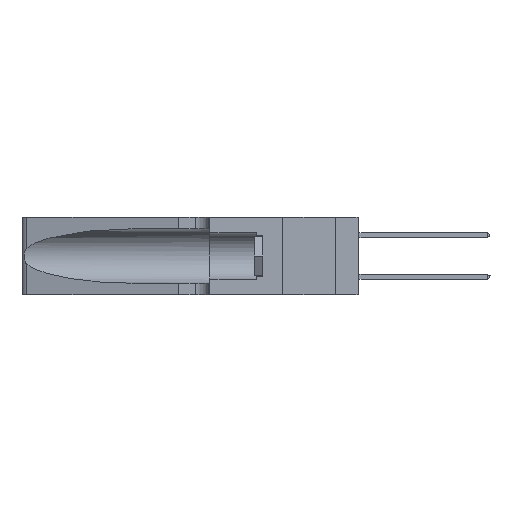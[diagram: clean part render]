
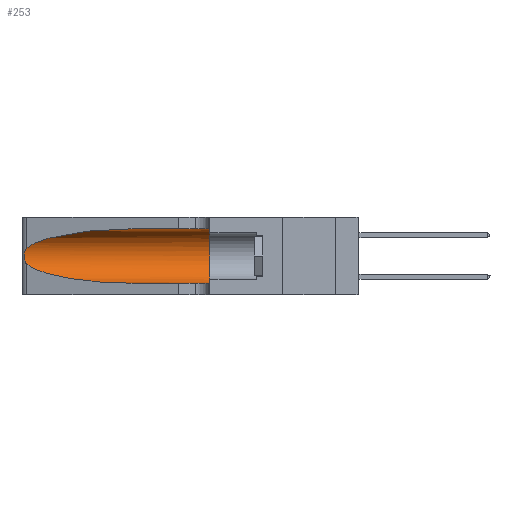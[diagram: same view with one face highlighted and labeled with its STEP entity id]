
A CAD part, left-side view. The second image highlights one B-rep face of the part: STEP entity #253.
In plain terms, the highlighted cylindrical face has radius 3.308 mm (diameter 6.617 mm), a partial arc.
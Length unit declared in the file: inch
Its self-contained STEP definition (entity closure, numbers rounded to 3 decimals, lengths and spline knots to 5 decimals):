
#198 = EDGE_CURVE ( 'NONE', #13411, #4651, #29645, .T. ) ;
#253 = ADVANCED_FACE ( 'NONE', ( #21866 ), #13304, .F. ) ;
#321 = DIRECTION ( 'NONE',  ( 0., 0., -1. ) ) ;
#993 = EDGE_CURVE ( 'NONE', #29057, #10696, #4352, .T. ) ;
#1692 = LINE ( 'NONE', #2280, #30447 ) ;
#2112 = CARTESIAN_POINT ( 'NONE',  ( 0.25487, 1.22718, 0.14631 ) ) ;
#2280 = CARTESIAN_POINT ( 'NONE',  ( 0.1305, 1.61858, 0.05475 ) ) ;
#2541 = CARTESIAN_POINT ( 'NONE',  ( 0.1305, 0.35, 0.185 ) ) ;
#2938 = VERTEX_POINT ( 'NONE', #15680 ) ;
#3268 =( BOUNDED_CURVE ( )  B_SPLINE_CURVE ( 3, ( #12375, #4944, #30703, #20521 ),
 .UNSPECIFIED., .F., .F. ) 
 B_SPLINE_CURVE_WITH_KNOTS ( ( 4, 4 ),
 ( 1.5708, 2.84003 ),
 .UNSPECIFIED. ) 
 CURVE ( )  GEOMETRIC_REPRESENTATION_ITEM ( )  RATIONAL_B_SPLINE_CURVE ( ( 1., 0.87, 0.87, 1. ) ) 
 REPRESENTATION_ITEM ( '' )  );
#4018 = ORIENTED_EDGE ( 'NONE', *, *, #198, .F. ) ;
#4308 = CARTESIAN_POINT ( 'NONE',  ( 0.1305, 0.72297, 0.05475 ) ) ;
#4352 = B_SPLINE_CURVE_WITH_KNOTS ( 'NONE', 3,
 ( #29398, #29007, #20638, #8054, #11064, #17375, #7347, #25163, #14851, #28022, #33294, #7217, #13134, #15459 ),
 .UNSPECIFIED., .F., .F.,
 ( 4, 2, 2, 2, 2, 2, 4 ),
 ( 0., 0.00027, 0.00053, 0.00107, 0.0016, 0.00187, 0.00214 ),
 .UNSPECIFIED. ) ;
#4651 = VERTEX_POINT ( 'NONE', #15916 ) ;
#4819 = DIRECTION ( 'NONE',  ( 0., -1., 0. ) ) ;
#4944 = CARTESIAN_POINT ( 'NONE',  ( 0.18966, 0.96281, 0.31525 ) ) ;
#4966 = DIRECTION ( 'NONE',  ( 0., 0., 1. ) ) ;
#5296 = CARTESIAN_POINT ( 'NONE',  ( 0.25487, 1.22718, 0.22369 ) ) ;
#5901 = EDGE_LOOP ( 'NONE', ( #16968, #30369, #29658, #20630, #4018, #18480 ) ) ;
#6521 = DIRECTION ( 'NONE',  ( 0., -1., 0. ) ) ;
#6953 = VERTEX_POINT ( 'NONE', #18798 ) ;
#7217 = CARTESIAN_POINT ( 'NONE',  ( 0.25639, 1.23186, 0.15144 ) ) ;
#7347 = CARTESIAN_POINT ( 'NONE',  ( 0.26075, 1.23896, 0.19203 ) ) ;
#7474 = EDGE_CURVE ( 'NONE', #6953, #29057, #3268, .T. ) ;
#8054 = CARTESIAN_POINT ( 'NONE',  ( 0.25787, 1.23484, 0.2124 ) ) ;
#8630 = CARTESIAN_POINT ( 'NONE',  ( 0.1305, 1.61858, 0.185 ) ) ;
#10174 = LINE ( 'NONE', #22243, #12628 ) ;
#10696 = VERTEX_POINT ( 'NONE', #2112 ) ;
#11064 = CARTESIAN_POINT ( 'NONE',  ( 0.25854, 1.2359, 0.20912 ) ) ;
#11968 = AXIS2_PLACEMENT_3D ( 'NONE', #2541, #12883, #4966 ) ;
#12375 = CARTESIAN_POINT ( 'NONE',  ( 0.1305, 0.72297, 0.31525 ) ) ;
#12628 = VECTOR ( 'NONE', #6521, 39.37008 ) ;
#12883 = DIRECTION ( 'NONE',  ( 0., 1., 0. ) ) ;
#13134 = CARTESIAN_POINT ( 'NONE',  ( 0.25555, 1.22993, 0.14849 ) ) ;
#13304 = CYLINDRICAL_SURFACE ( 'NONE', #29947, 0.13025 ) ;
#13411 = VERTEX_POINT ( 'NONE', #27493 ) ;
#14508 = EDGE_CURVE ( 'NONE', #10696, #2938, #22195, .T. ) ;
#14851 = CARTESIAN_POINT ( 'NONE',  ( 0.26017, 1.23833, 0.17102 ) ) ;
#15459 = CARTESIAN_POINT ( 'NONE',  ( 0.25487, 1.22718, 0.14631 ) ) ;
#15680 = CARTESIAN_POINT ( 'NONE',  ( 0.1305, 0.72297, 0.05475 ) ) ;
#15916 = CARTESIAN_POINT ( 'NONE',  ( 0.1305, 0.35, 0.05475 ) ) ;
#16550 = EDGE_CURVE ( 'NONE', #6953, #13411, #10174, .T. ) ;
#16798 = CARTESIAN_POINT ( 'NONE',  ( 0.25487, 1.22718, 0.14631 ) ) ;
#16968 = ORIENTED_EDGE ( 'NONE', *, *, #7474, .T. ) ;
#17375 = CARTESIAN_POINT ( 'NONE',  ( 0.26018, 1.23835, 0.19895 ) ) ;
#18480 = ORIENTED_EDGE ( 'NONE', *, *, #16550, .F. ) ;
#18798 = CARTESIAN_POINT ( 'NONE',  ( 0.1305, 0.72297, 0.31525 ) ) ;
#20521 = CARTESIAN_POINT ( 'NONE',  ( 0.25487, 1.22718, 0.22369 ) ) ;
#20630 = ORIENTED_EDGE ( 'NONE', *, *, #26491, .T. ) ;
#20638 = CARTESIAN_POINT ( 'NONE',  ( 0.25639, 1.23184, 0.21858 ) ) ;
#21866 = FACE_OUTER_BOUND ( 'NONE', #5901, .T. ) ;
#22195 =( BOUNDED_CURVE ( )  B_SPLINE_CURVE ( 3, ( #16798, #24346, #30562, #4308 ),
 .UNSPECIFIED., .F., .F. ) 
 B_SPLINE_CURVE_WITH_KNOTS ( ( 4, 4 ),
 ( 3.44316, 4.71239 ),
 .UNSPECIFIED. ) 
 CURVE ( )  GEOMETRIC_REPRESENTATION_ITEM ( )  RATIONAL_B_SPLINE_CURVE ( ( 1., 0.87, 0.87, 1. ) ) 
 REPRESENTATION_ITEM ( '' )  );
#22243 = CARTESIAN_POINT ( 'NONE',  ( 0.1305, 1.61858, 0.31525 ) ) ;
#23882 = DIRECTION ( 'NONE',  ( 0., -1., 0. ) ) ;
#24346 = CARTESIAN_POINT ( 'NONE',  ( 0.2373, 1.15595, 0.08982 ) ) ;
#25163 = CARTESIAN_POINT ( 'NONE',  ( 0.26075, 1.23896, 0.178 ) ) ;
#26491 = EDGE_CURVE ( 'NONE', #2938, #4651, #1692, .T. ) ;
#27493 = CARTESIAN_POINT ( 'NONE',  ( 0.1305, 0.35, 0.31525 ) ) ;
#28022 = CARTESIAN_POINT ( 'NONE',  ( 0.25856, 1.23593, 0.16098 ) ) ;
#29007 = CARTESIAN_POINT ( 'NONE',  ( 0.25555, 1.22994, 0.2215 ) ) ;
#29057 = VERTEX_POINT ( 'NONE', #5296 ) ;
#29398 = CARTESIAN_POINT ( 'NONE',  ( 0.25487, 1.22718, 0.22369 ) ) ;
#29645 = CIRCLE ( 'NONE', #11968, 0.13025 ) ;
#29658 = ORIENTED_EDGE ( 'NONE', *, *, #14508, .T. ) ;
#29947 = AXIS2_PLACEMENT_3D ( 'NONE', #8630, #23882, #321 ) ;
#30369 = ORIENTED_EDGE ( 'NONE', *, *, #993, .T. ) ;
#30447 = VECTOR ( 'NONE', #4819, 39.37008 ) ;
#30562 = CARTESIAN_POINT ( 'NONE',  ( 0.18966, 0.96281, 0.05475 ) ) ;
#30703 = CARTESIAN_POINT ( 'NONE',  ( 0.2373, 1.15595, 0.28018 ) ) ;
#33294 = CARTESIAN_POINT ( 'NONE',  ( 0.25789, 1.23486, 0.15765 ) ) ;
